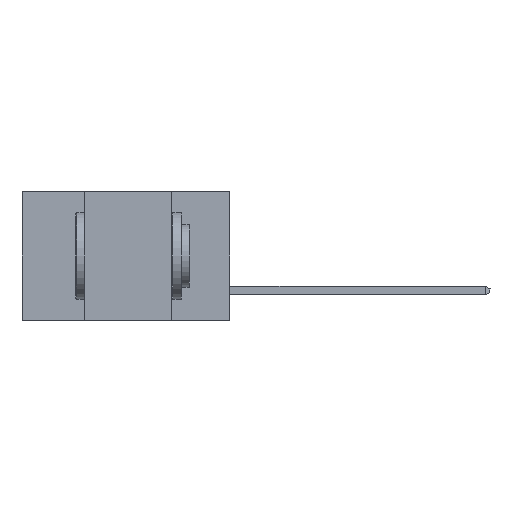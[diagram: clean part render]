
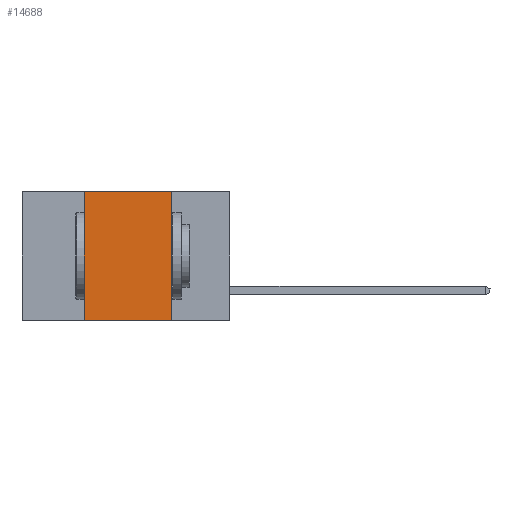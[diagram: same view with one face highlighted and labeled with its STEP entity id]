
A CAD part, left-side view. The second image highlights one B-rep face of the part: STEP entity #14688.
In plain terms, the highlighted planar face has unit normal (-1, 0, 0).
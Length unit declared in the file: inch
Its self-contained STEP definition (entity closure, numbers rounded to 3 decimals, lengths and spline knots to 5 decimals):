
#482 = EDGE_CURVE ( 'NONE', #19826, #3226, #5266, .T. ) ;
#510 = VERTEX_POINT ( 'NONE', #25516 ) ;
#952 = CARTESIAN_POINT ( 'NONE',  ( 0., 0.6, 0. ) ) ;
#1529 = VECTOR ( 'NONE', #18731, 39.37008 ) ;
#1759 = AXIS2_PLACEMENT_3D ( 'NONE', #16454, #24553, #14855 ) ;
#2975 = EDGE_CURVE ( 'NONE', #4135, #510, #4770, .T. ) ;
#3226 = VERTEX_POINT ( 'NONE', #6083 ) ;
#4135 = VERTEX_POINT ( 'NONE', #8933 ) ;
#4770 = LINE ( 'NONE', #25279, #11638 ) ;
#5266 = LINE ( 'NONE', #7805, #11623 ) ;
#6083 = CARTESIAN_POINT ( 'NONE',  ( 0., 0.17, -0.37 ) ) ;
#7805 = CARTESIAN_POINT ( 'NONE',  ( 0., 0.17, -0.37 ) ) ;
#7941 = VECTOR ( 'NONE', #11075, 39.37008 ) ;
#8933 = CARTESIAN_POINT ( 'NONE',  ( 0., 0.42, -0.37 ) ) ;
#9318 = DIRECTION ( 'NONE',  ( 0., 0., 1. ) ) ;
#9561 = CARTESIAN_POINT ( 'NONE',  ( 0., 0.17, 0. ) ) ;
#10332 = LINE ( 'NONE', #20328, #1529 ) ;
#11075 = DIRECTION ( 'NONE',  ( 0., -1., 0. ) ) ;
#11320 = EDGE_LOOP ( 'NONE', ( #24542, #12530, #13302, #23547 ) ) ;
#11623 = VECTOR ( 'NONE', #21529, 39.37008 ) ;
#11638 = VECTOR ( 'NONE', #9318, 39.37008 ) ;
#12530 = ORIENTED_EDGE ( 'NONE', *, *, #22541, .F. ) ;
#13302 = ORIENTED_EDGE ( 'NONE', *, *, #2975, .F. ) ;
#14688 = ADVANCED_FACE ( 'NONE', ( #18572 ), #20703, .F. ) ;
#14855 = DIRECTION ( 'NONE',  ( 0., 0., -1. ) ) ;
#16454 = CARTESIAN_POINT ( 'NONE',  ( 0., 0.6, 0. ) ) ;
#17486 = LINE ( 'NONE', #952, #7941 ) ;
#18572 = FACE_OUTER_BOUND ( 'NONE', #11320, .T. ) ;
#18731 = DIRECTION ( 'NONE',  ( 0., -1., 0. ) ) ;
#19826 = VERTEX_POINT ( 'NONE', #9561 ) ;
#20328 = CARTESIAN_POINT ( 'NONE',  ( 0., 0.6, -0.37 ) ) ;
#20703 = PLANE ( 'NONE',  #1759 ) ;
#21529 = DIRECTION ( 'NONE',  ( 0., 0., -1. ) ) ;
#22541 = EDGE_CURVE ( 'NONE', #510, #19826, #17486, .T. ) ;
#23547 = ORIENTED_EDGE ( 'NONE', *, *, #24881, .T. ) ;
#24542 = ORIENTED_EDGE ( 'NONE', *, *, #482, .F. ) ;
#24553 = DIRECTION ( 'NONE',  ( 1., 0., 0. ) ) ;
#24881 = EDGE_CURVE ( 'NONE', #4135, #3226, #10332, .T. ) ;
#25279 = CARTESIAN_POINT ( 'NONE',  ( 0., 0.42, -0.37 ) ) ;
#25516 = CARTESIAN_POINT ( 'NONE',  ( 0., 0.42, 0. ) ) ;
